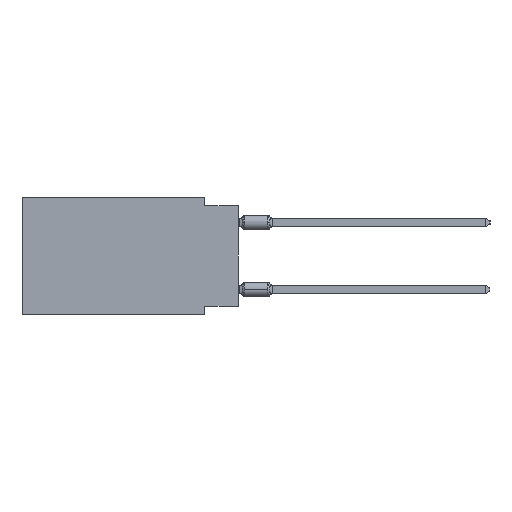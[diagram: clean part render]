
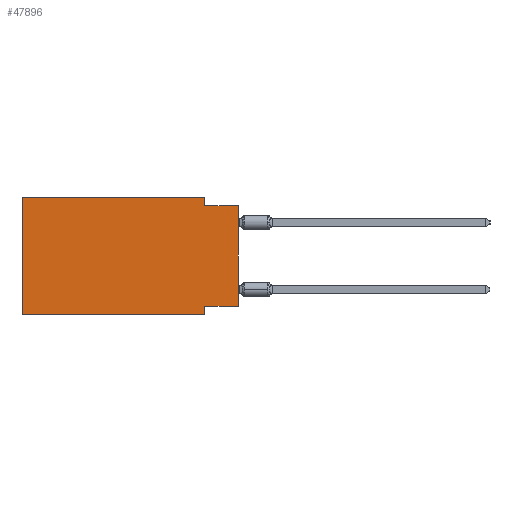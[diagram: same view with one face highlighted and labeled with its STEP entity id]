
A CAD part, left-side view. The second image highlights one B-rep face of the part: STEP entity #47896.
In plain terms, the highlighted planar face has unit normal (-1, 0, 0).
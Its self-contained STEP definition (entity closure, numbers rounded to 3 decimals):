
#897 = LINE ( 'NONE', #22149, #1592 ) ;
#1592 = VECTOR ( 'NONE', #54195, 1000. ) ;
#4411 = ORIENTED_EDGE ( 'NONE', *, *, #42621, .F. ) ;
#4818 = CARTESIAN_POINT ( 'NONE',  ( 0., 16.383, 0. ) ) ;
#5595 = VECTOR ( 'NONE', #21388, 1000. ) ;
#5840 = ORIENTED_EDGE ( 'NONE', *, *, #40451, .F. ) ;
#6375 = CARTESIAN_POINT ( 'NONE',  ( 0., 16.383, 0. ) ) ;
#7767 = LINE ( 'NONE', #45055, #66344 ) ;
#8646 = CARTESIAN_POINT ( 'NONE',  ( 0., 16.383, 0. ) ) ;
#12296 = CARTESIAN_POINT ( 'NONE',  ( 0., 0., -0.635 ) ) ;
#13455 = LINE ( 'NONE', #24262, #38557 ) ;
#13514 = LINE ( 'NONE', #40335, #60390 ) ;
#17962 = AXIS2_PLACEMENT_3D ( 'NONE', #8646, #55712, #19108 ) ;
#19108 = DIRECTION ( 'NONE',  ( 0., 0., -1. ) ) ;
#20126 = CARTESIAN_POINT ( 'NONE',  ( 0., 16.383, -8.89 ) ) ;
#21388 = DIRECTION ( 'NONE',  ( 0., 0., 1. ) ) ;
#22083 = CARTESIAN_POINT ( 'NONE',  ( 0., 0., 0. ) ) ;
#22149 = CARTESIAN_POINT ( 'NONE',  ( 0., 0., -8.255 ) ) ;
#22482 = EDGE_CURVE ( 'NONE', #31936, #32682, #13514, .T. ) ;
#23449 = VERTEX_POINT ( 'NONE', #20126 ) ;
#24262 = CARTESIAN_POINT ( 'NONE',  ( 0., 2.54, -8.89 ) ) ;
#24646 = CARTESIAN_POINT ( 'NONE',  ( 0., 0., -8.255 ) ) ;
#24705 = LINE ( 'NONE', #45964, #35921 ) ;
#25616 = EDGE_CURVE ( 'NONE', #23449, #48227, #7767, .T. ) ;
#28992 = VECTOR ( 'NONE', #37899, 1000. ) ;
#29979 = EDGE_CURVE ( 'NONE', #33005, #35604, #52749, .T. ) ;
#31936 = VERTEX_POINT ( 'NONE', #63633 ) ;
#32450 = EDGE_LOOP ( 'NONE', ( #56377, #37029, #49648, #4411, #41666, #51979, #34066, #5840 ) ) ;
#32646 = VECTOR ( 'NONE', #32790, 1000. ) ;
#32682 = VERTEX_POINT ( 'NONE', #47352 ) ;
#32790 = DIRECTION ( 'NONE',  ( 0., 0., 1. ) ) ;
#33005 = VERTEX_POINT ( 'NONE', #24646 ) ;
#34066 = ORIENTED_EDGE ( 'NONE', *, *, #66920, .F. ) ;
#34703 = CARTESIAN_POINT ( 'NONE',  ( 0., 2.54, -8.255 ) ) ;
#34793 = DIRECTION ( 'NONE',  ( 0., 0., -1. ) ) ;
#35604 = VERTEX_POINT ( 'NONE', #12296 ) ;
#35921 = VECTOR ( 'NONE', #62003, 1000. ) ;
#37029 = ORIENTED_EDGE ( 'NONE', *, *, #37919, .F. ) ;
#37899 = DIRECTION ( 'NONE',  ( 0., -1., 0. ) ) ;
#37919 = EDGE_CURVE ( 'NONE', #32682, #35604, #24705, .T. ) ;
#38227 = CARTESIAN_POINT ( 'NONE',  ( 0., 2.54, -8.89 ) ) ;
#38557 = VECTOR ( 'NONE', #57360, 1000. ) ;
#38786 = EDGE_CURVE ( 'NONE', #23449, #45001, #58235, .T. ) ;
#40335 = CARTESIAN_POINT ( 'NONE',  ( 0., 2.54, 0. ) ) ;
#40451 = EDGE_CURVE ( 'NONE', #33005, #64402, #897, .T. ) ;
#41051 = PLANE ( 'NONE',  #17962 ) ;
#41666 = ORIENTED_EDGE ( 'NONE', *, *, #38786, .F. ) ;
#42621 = EDGE_CURVE ( 'NONE', #45001, #31936, #54381, .T. ) ;
#45001 = VERTEX_POINT ( 'NONE', #6375 ) ;
#45055 = CARTESIAN_POINT ( 'NONE',  ( 0., 16.383, -8.89 ) ) ;
#45248 = FACE_OUTER_BOUND ( 'NONE', #32450, .T. ) ;
#45964 = CARTESIAN_POINT ( 'NONE',  ( 0., 0., -0.635 ) ) ;
#47352 = CARTESIAN_POINT ( 'NONE',  ( 0., 2.54, -0.635 ) ) ;
#47896 = ADVANCED_FACE ( 'NONE', ( #45248 ), #41051, .F. ) ;
#48227 = VERTEX_POINT ( 'NONE', #38227 ) ;
#49648 = ORIENTED_EDGE ( 'NONE', *, *, #22482, .F. ) ;
#51979 = ORIENTED_EDGE ( 'NONE', *, *, #25616, .T. ) ;
#52749 = LINE ( 'NONE', #22083, #5595 ) ;
#52991 = CARTESIAN_POINT ( 'NONE',  ( 0., 16.383, 0. ) ) ;
#54195 = DIRECTION ( 'NONE',  ( 0., 1., 0. ) ) ;
#54381 = LINE ( 'NONE', #4818, #28992 ) ;
#55712 = DIRECTION ( 'NONE',  ( 1., 0., 0. ) ) ;
#56377 = ORIENTED_EDGE ( 'NONE', *, *, #29979, .T. ) ;
#57360 = DIRECTION ( 'NONE',  ( 0., 0., -1. ) ) ;
#58235 = LINE ( 'NONE', #52991, #32646 ) ;
#60390 = VECTOR ( 'NONE', #34793, 1000. ) ;
#61082 = DIRECTION ( 'NONE',  ( 0., -1., 0. ) ) ;
#62003 = DIRECTION ( 'NONE',  ( 0., -1., 0. ) ) ;
#63633 = CARTESIAN_POINT ( 'NONE',  ( 0., 2.54, 0. ) ) ;
#64402 = VERTEX_POINT ( 'NONE', #34703 ) ;
#66344 = VECTOR ( 'NONE', #61082, 1000. ) ;
#66920 = EDGE_CURVE ( 'NONE', #64402, #48227, #13455, .T. ) ;
